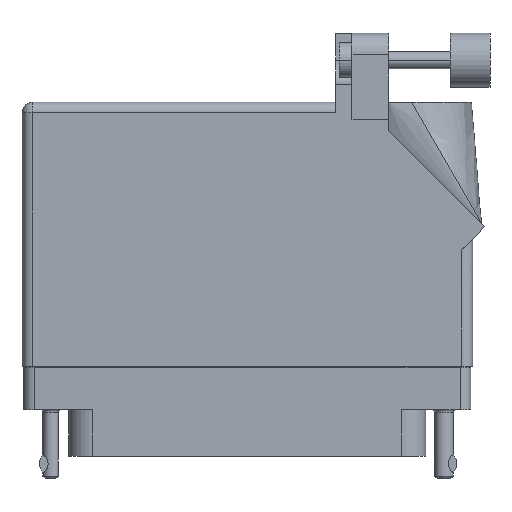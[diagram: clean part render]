
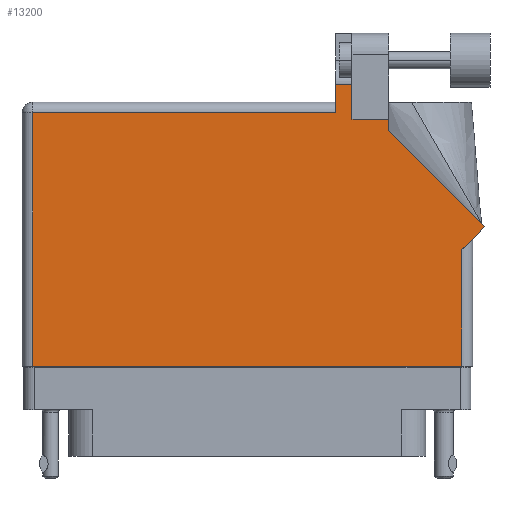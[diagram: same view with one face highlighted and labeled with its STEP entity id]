
A CAD part, front view. The second image highlights one B-rep face of the part: STEP entity #13200.
In plain terms, the highlighted face is planar.
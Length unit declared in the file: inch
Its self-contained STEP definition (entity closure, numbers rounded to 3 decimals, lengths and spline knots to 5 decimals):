
#2073 = VERTEX_POINT ( 'NONE', #33268 ) ;
#2393 = CARTESIAN_POINT ( 'NONE',  ( 0.82, 1.26442, 0.455 ) ) ;
#3328 = VECTOR ( 'NONE', #58774, 39.37008 ) ;
#3849 = CARTESIAN_POINT ( 'NONE',  ( 0.513, 1.368, 0.455 ) ) ;
#3980 = CARTESIAN_POINT ( 'NONE',  ( -1.306, 1.368, 0.455 ) ) ;
#4017 = EDGE_CURVE ( 'NONE', #47714, #16094, #39989, .T. ) ;
#4298 = DIRECTION ( 'NONE',  ( 0., 1., 0. ) ) ;
#4815 = CARTESIAN_POINT ( 'NONE',  ( 1.306, 0.637, 0.455 ) ) ;
#6220 = VERTEX_POINT ( 'NONE', #30685 ) ;
#6802 = CARTESIAN_POINT ( 'NONE',  ( -1.244, -0.1, 0.455 ) ) ;
#7905 = AXIS2_PLACEMENT_3D ( 'NONE', #41813, #51355, #51147 ) ;
#8425 = PLANE ( 'NONE',  #7905 ) ;
#8636 = LINE ( 'NONE', #21430, #36807 ) ;
#9593 = LINE ( 'NONE', #14753, #27372 ) ;
#9639 = EDGE_CURVE ( 'NONE', #43131, #10175, #33707, .T. ) ;
#9911 = EDGE_LOOP ( 'NONE', ( #14010, #30532, #20371, #58541, #42108, #54028, #20605, #50216, #16874, #24943, #59827 ) ) ;
#10175 = VERTEX_POINT ( 'NONE', #37458 ) ;
#10533 = CARTESIAN_POINT ( 'NONE',  ( 0.513, 1.5315, 0.455 ) ) ;
#11286 = VECTOR ( 'NONE', #58913, 39.37008 ) ;
#11348 = VECTOR ( 'NONE', #52326, 39.37008 ) ;
#12145 = VERTEX_POINT ( 'NONE', #3849 ) ;
#13200 = ADVANCED_FACE ( 'NONE', ( #29671 ), #8425, .F. ) ;
#14010 = ORIENTED_EDGE ( 'NONE', *, *, #32978, .T. ) ;
#14753 = CARTESIAN_POINT ( 'NONE',  ( 0.513, 1.43, 0.455 ) ) ;
#16094 = VERTEX_POINT ( 'NONE', #10533 ) ;
#16874 = ORIENTED_EDGE ( 'NONE', *, *, #21845, .T. ) ;
#16992 = CARTESIAN_POINT ( 'NONE',  ( 0.607, 1.5315, 0.455 ) ) ;
#20371 = ORIENTED_EDGE ( 'NONE', *, *, #28789, .T. ) ;
#20605 = ORIENTED_EDGE ( 'NONE', *, *, #54433, .T. ) ;
#21430 = CARTESIAN_POINT ( 'NONE',  ( 0.82, 1.33, 0.455 ) ) ;
#21845 = EDGE_CURVE ( 'NONE', #45658, #27593, #53557, .T. ) ;
#23219 = LINE ( 'NONE', #3980, #11348 ) ;
#23814 = VECTOR ( 'NONE', #26623, 39.37008 ) ;
#24525 = LINE ( 'NONE', #54974, #23814 ) ;
#24659 = DIRECTION ( 'NONE',  ( 0., -1., 0. ) ) ;
#24943 = ORIENTED_EDGE ( 'NONE', *, *, #47510, .T. ) ;
#26623 = DIRECTION ( 'NONE',  ( 0., -1., 0. ) ) ;
#27266 = VECTOR ( 'NONE', #46702, 39.37008 ) ;
#27372 = VECTOR ( 'NONE', #24659, 39.37008 ) ;
#27373 = VECTOR ( 'NONE', #33501, 39.37008 ) ;
#27593 = VERTEX_POINT ( 'NONE', #45115 ) ;
#28789 = EDGE_CURVE ( 'NONE', #16094, #12145, #9593, .T. ) ;
#29671 = FACE_OUTER_BOUND ( 'NONE', #9911, .T. ) ;
#30038 = EDGE_CURVE ( 'NONE', #35001, #60443, #8636, .T. ) ;
#30048 = LINE ( 'NONE', #4815, #32226 ) ;
#30306 = CARTESIAN_POINT ( 'NONE',  ( 1.37671, 0.70771, 0.455 ) ) ;
#30532 = ORIENTED_EDGE ( 'NONE', *, *, #4017, .T. ) ;
#30685 = CARTESIAN_POINT ( 'NONE',  ( -1.244, 1.368, 0.455 ) ) ;
#30761 = DIRECTION ( 'NONE',  ( 1., 0., 0. ) ) ;
#30948 = DIRECTION ( 'NONE',  ( -1., 0., 0. ) ) ;
#32023 = LINE ( 'NONE', #42067, #59476 ) ;
#32226 = VECTOR ( 'NONE', #37987, 39.37008 ) ;
#32978 = EDGE_CURVE ( 'NONE', #60443, #47714, #36865, .T. ) ;
#33056 = LINE ( 'NONE', #2393, #3328 ) ;
#33268 = CARTESIAN_POINT ( 'NONE',  ( 1.244, 0.575, 0.455 ) ) ;
#33501 = DIRECTION ( 'NONE',  ( -1., 0., 0. ) ) ;
#33707 = LINE ( 'NONE', #58906, #59584 ) ;
#35001 = VERTEX_POINT ( 'NONE', #54133 ) ;
#36807 = VECTOR ( 'NONE', #30948, 39.37008 ) ;
#36865 = LINE ( 'NONE', #46100, #27266 ) ;
#37444 = CARTESIAN_POINT ( 'NONE',  ( 0.93777, 1.5315, 0.455 ) ) ;
#37458 = CARTESIAN_POINT ( 'NONE',  ( 1.244, -0.1, 0.455 ) ) ;
#37987 = DIRECTION ( 'NONE',  ( 0.707, 0.707, 0. ) ) ;
#39989 = LINE ( 'NONE', #37444, #27373 ) ;
#41813 = CARTESIAN_POINT ( 'NONE',  ( -1.306, 1.43, 0.455 ) ) ;
#42067 = CARTESIAN_POINT ( 'NONE',  ( 1.244, 0.637, 0.455 ) ) ;
#42108 = ORIENTED_EDGE ( 'NONE', *, *, #56287, .T. ) ;
#42968 = EDGE_CURVE ( 'NONE', #2073, #45658, #30048, .T. ) ;
#43131 = VERTEX_POINT ( 'NONE', #6802 ) ;
#45079 = CARTESIAN_POINT ( 'NONE',  ( 1.37671, 0.70771, 0.455 ) ) ;
#45115 = CARTESIAN_POINT ( 'NONE',  ( 0.82, 1.26442, 0.455 ) ) ;
#45163 = EDGE_CURVE ( 'NONE', #12145, #6220, #23219, .T. ) ;
#45658 = VERTEX_POINT ( 'NONE', #30306 ) ;
#46100 = CARTESIAN_POINT ( 'NONE',  ( 0.607, 1.33, 0.455 ) ) ;
#46702 = DIRECTION ( 'NONE',  ( 0., 1., 0. ) ) ;
#47510 = EDGE_CURVE ( 'NONE', #27593, #35001, #33056, .T. ) ;
#47714 = VERTEX_POINT ( 'NONE', #16992 ) ;
#50216 = ORIENTED_EDGE ( 'NONE', *, *, #42968, .T. ) ;
#51147 = DIRECTION ( 'NONE',  ( -1., 0., 0. ) ) ;
#51355 = DIRECTION ( 'NONE',  ( 0., 0., -1. ) ) ;
#52326 = DIRECTION ( 'NONE',  ( -1., 0., 0. ) ) ;
#53306 = CARTESIAN_POINT ( 'NONE',  ( 0.607, 1.33, 0.455 ) ) ;
#53557 = LINE ( 'NONE', #45079, #11286 ) ;
#54028 = ORIENTED_EDGE ( 'NONE', *, *, #9639, .T. ) ;
#54133 = CARTESIAN_POINT ( 'NONE',  ( 0.82, 1.33, 0.455 ) ) ;
#54433 = EDGE_CURVE ( 'NONE', #10175, #2073, #32023, .T. ) ;
#54974 = CARTESIAN_POINT ( 'NONE',  ( -1.244, -0.1, 0.455 ) ) ;
#56287 = EDGE_CURVE ( 'NONE', #6220, #43131, #24525, .T. ) ;
#58541 = ORIENTED_EDGE ( 'NONE', *, *, #45163, .T. ) ;
#58774 = DIRECTION ( 'NONE',  ( 0., 1., 0. ) ) ;
#58906 = CARTESIAN_POINT ( 'NONE',  ( -1.306, -0.1, 0.455 ) ) ;
#58913 = DIRECTION ( 'NONE',  ( -0.707, 0.707, 0. ) ) ;
#59476 = VECTOR ( 'NONE', #4298, 39.37008 ) ;
#59584 = VECTOR ( 'NONE', #30761, 39.37008 ) ;
#59827 = ORIENTED_EDGE ( 'NONE', *, *, #30038, .T. ) ;
#60443 = VERTEX_POINT ( 'NONE', #53306 ) ;
